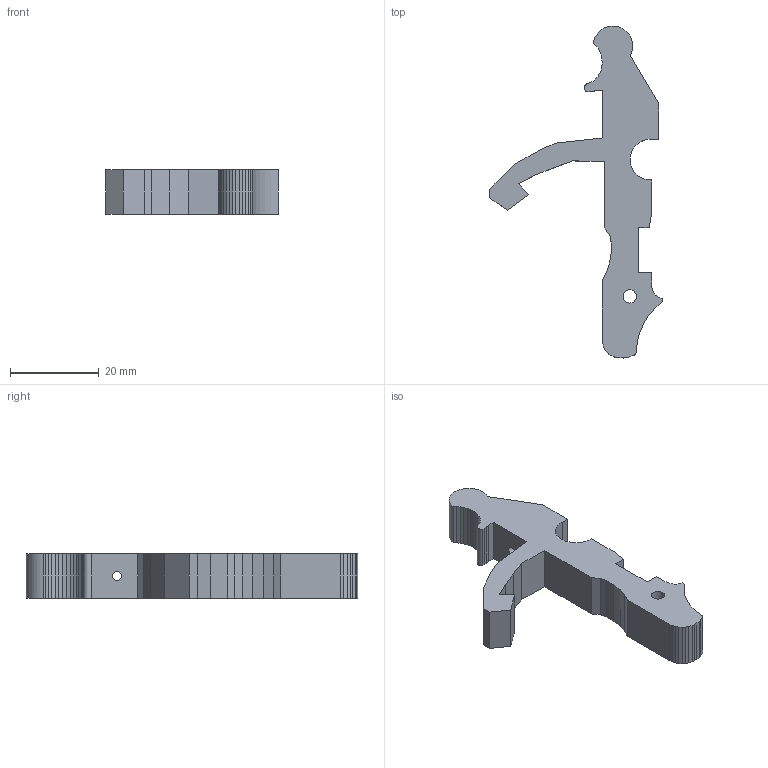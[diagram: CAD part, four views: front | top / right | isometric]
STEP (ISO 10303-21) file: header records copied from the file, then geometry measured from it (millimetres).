
FILE_DESCRIPTION((''),'2;1');
FILE_NAME('hammer.stp','2013-08-15T20:11:54',('mrfr'),(''),'Autodesk Inventor 2013','Autodesk Inventor 2013','');
FILE_SCHEMA(('AUTOMOTIVE_DESIGN { 1 0 10303 214 1 1 1 1 }'));
Length unit declared in the file: millimetre
Products named in the file (1): hammer
Bounding box: 38.8 x 74.71 x 10 mm (x, y, z)
Volume: 8253.4 mm3; surface area: 4275.9 mm2
Topology: 1 solids, 1 shells, 79 faces, 231 edges, 154 vertices
Faces by surface type: plane 72, cylinder 7
Full cylindrical faces by diameter (mm): 2 x1, 3 x1
Entity records: 2603 total; most frequent: CARTESIAN_POINT 463, ORIENTED_EDGE 458, DIRECTION 403, EDGE_CURVE 229, VECTOR 215, LINE 215, VERTEX_POINT 154, AXIS2_PLACEMENT_3D 94
